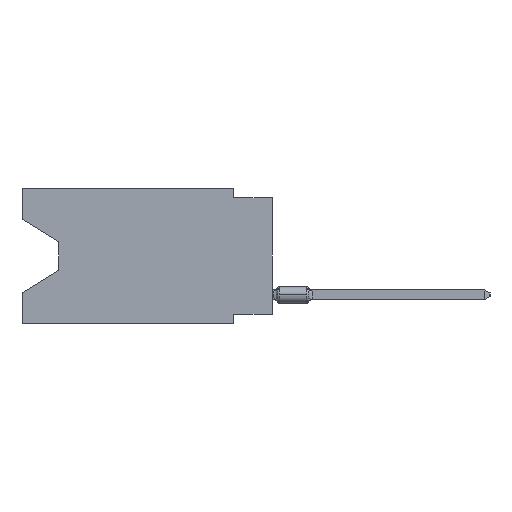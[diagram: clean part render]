
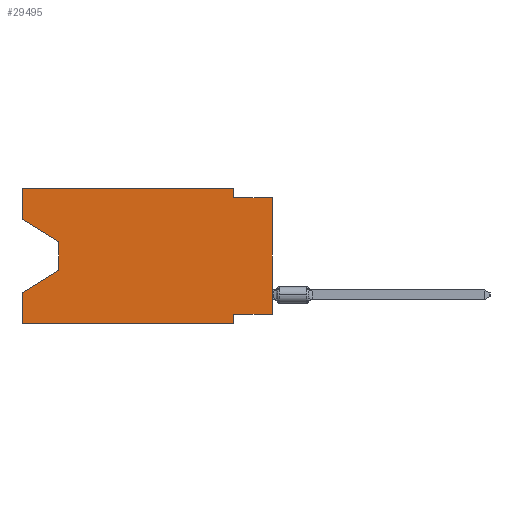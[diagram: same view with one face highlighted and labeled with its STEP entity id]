
A CAD part, left-side view. The second image highlights one B-rep face of the part: STEP entity #29495.
In plain terms, the highlighted planar face has unit normal (-1, 0, 0).
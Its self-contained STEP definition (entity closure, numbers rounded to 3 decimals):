
#459 = LINE ( 'NONE', #22005, #38883 ) ;
#727 = EDGE_CURVE ( 'NONE', #10351, #27550, #41165, .T. ) ;
#1693 = CARTESIAN_POINT ( 'NONE',  ( 0., 0., -0.635 ) ) ;
#2124 = ORIENTED_EDGE ( 'NONE', *, *, #29716, .F. ) ;
#2847 = DIRECTION ( 'NONE',  ( 0., 0., -1. ) ) ;
#3180 = DIRECTION ( 'NONE',  ( 0., -1., 0. ) ) ;
#3705 = EDGE_CURVE ( 'NONE', #16135, #55146, #459, .T. ) ;
#4268 = DIRECTION ( 'NONE',  ( 0., 0., 1. ) ) ;
#4366 = ORIENTED_EDGE ( 'NONE', *, *, #41531, .F. ) ;
#4495 = EDGE_CURVE ( 'NONE', #27789, #14697, #29705, .T. ) ;
#5082 = DIRECTION ( 'NONE',  ( 0., 0., 1. ) ) ;
#6002 = CARTESIAN_POINT ( 'NONE',  ( 0., 16.383, -2.038 ) ) ;
#6176 = DIRECTION ( 'NONE',  ( 0., -1., 0. ) ) ;
#6498 = VERTEX_POINT ( 'NONE', #50728 ) ;
#7904 = CARTESIAN_POINT ( 'NONE',  ( 0., 0., 0. ) ) ;
#8029 = CARTESIAN_POINT ( 'NONE',  ( 0., 16.383, 0. ) ) ;
#8824 = LINE ( 'NONE', #26709, #41561 ) ;
#9826 = VERTEX_POINT ( 'NONE', #49475 ) ;
#10351 = VERTEX_POINT ( 'NONE', #53186 ) ;
#11105 = EDGE_CURVE ( 'NONE', #41352, #16135, #35303, .T. ) ;
#13425 = EDGE_CURVE ( 'NONE', #32368, #14697, #52826, .T. ) ;
#14277 = CARTESIAN_POINT ( 'NONE',  ( 0., 16.383, 0. ) ) ;
#14690 = CARTESIAN_POINT ( 'NONE',  ( 0., 16.383, -8.89 ) ) ;
#14697 = VERTEX_POINT ( 'NONE', #53657 ) ;
#15270 = EDGE_CURVE ( 'NONE', #44979, #41352, #35899, .T. ) ;
#15278 = VECTOR ( 'NONE', #31653, 1000. ) ;
#15598 = LINE ( 'NONE', #8029, #26153 ) ;
#15712 = CARTESIAN_POINT ( 'NONE',  ( 0., 2.54, -8.89 ) ) ;
#16135 = VERTEX_POINT ( 'NONE', #48827 ) ;
#16492 = VECTOR ( 'NONE', #44002, 1000. ) ;
#16639 = EDGE_CURVE ( 'NONE', #6498, #9826, #49581, .T. ) ;
#17535 = DIRECTION ( 'NONE',  ( 0., 0.855, -0.519 ) ) ;
#18446 = PLANE ( 'NONE',  #30715 ) ;
#19275 = DIRECTION ( 'NONE',  ( 1., 0., 0. ) ) ;
#19652 = ORIENTED_EDGE ( 'NONE', *, *, #13425, .F. ) ;
#22005 = CARTESIAN_POINT ( 'NONE',  ( 0., 13.97, -5.385 ) ) ;
#23221 = LINE ( 'NONE', #27414, #32297 ) ;
#25276 = ORIENTED_EDGE ( 'NONE', *, *, #4495, .T. ) ;
#26149 = DIRECTION ( 'NONE',  ( 0., 1., 0. ) ) ;
#26153 = VECTOR ( 'NONE', #30390, 1000. ) ;
#26158 = CARTESIAN_POINT ( 'NONE',  ( 0., 16.383, -6.852 ) ) ;
#26709 = CARTESIAN_POINT ( 'NONE',  ( 0., 0., -8.255 ) ) ;
#27172 = VERTEX_POINT ( 'NONE', #50651 ) ;
#27414 = CARTESIAN_POINT ( 'NONE',  ( 0., 2.54, 0. ) ) ;
#27550 = VERTEX_POINT ( 'NONE', #37206 ) ;
#27644 = FACE_OUTER_BOUND ( 'NONE', #46805, .T. ) ;
#27789 = VERTEX_POINT ( 'NONE', #36030 ) ;
#29495 = ADVANCED_FACE ( 'NONE', ( #27644 ), #18446, .F. ) ;
#29705 = LINE ( 'NONE', #7904, #40766 ) ;
#29716 = EDGE_CURVE ( 'NONE', #44979, #6498, #15598, .T. ) ;
#30390 = DIRECTION ( 'NONE',  ( 0., 0., 1. ) ) ;
#30715 = AXIS2_PLACEMENT_3D ( 'NONE', #44951, #19275, #35748 ) ;
#31315 = LINE ( 'NONE', #14277, #38587 ) ;
#31653 = DIRECTION ( 'NONE',  ( 0., 0., -1. ) ) ;
#31728 = DIRECTION ( 'NONE',  ( 0., -1., 0. ) ) ;
#32297 = VECTOR ( 'NONE', #44177, 1000. ) ;
#32368 = VERTEX_POINT ( 'NONE', #46707 ) ;
#33383 = VECTOR ( 'NONE', #2847, 1000. ) ;
#35040 = ORIENTED_EDGE ( 'NONE', *, *, #15270, .T. ) ;
#35303 = LINE ( 'NONE', #52060, #15278 ) ;
#35748 = DIRECTION ( 'NONE',  ( 0., 0., -1. ) ) ;
#35899 = LINE ( 'NONE', #6002, #16492 ) ;
#36030 = CARTESIAN_POINT ( 'NONE',  ( 0., 0., -8.255 ) ) ;
#36966 = ORIENTED_EDGE ( 'NONE', *, *, #37286, .T. ) ;
#37081 = ORIENTED_EDGE ( 'NONE', *, *, #16639, .F. ) ;
#37206 = CARTESIAN_POINT ( 'NONE',  ( 0., 2.54, -8.89 ) ) ;
#37286 = EDGE_CURVE ( 'NONE', #27172, #27550, #52958, .T. ) ;
#38587 = VECTOR ( 'NONE', #5082, 1000. ) ;
#38883 = VECTOR ( 'NONE', #17535, 1000. ) ;
#39268 = VECTOR ( 'NONE', #31728, 1000. ) ;
#39593 = VECTOR ( 'NONE', #6176, 1000. ) ;
#40625 = ORIENTED_EDGE ( 'NONE', *, *, #727, .F. ) ;
#40766 = VECTOR ( 'NONE', #4268, 1000. ) ;
#41165 = LINE ( 'NONE', #15712, #33383 ) ;
#41352 = VERTEX_POINT ( 'NONE', #51459 ) ;
#41515 = EDGE_CURVE ( 'NONE', #27172, #55146, #31315, .T. ) ;
#41531 = EDGE_CURVE ( 'NONE', #9826, #32368, #23221, .T. ) ;
#41561 = VECTOR ( 'NONE', #26149, 1000. ) ;
#41757 = ORIENTED_EDGE ( 'NONE', *, *, #3705, .T. ) ;
#44002 = DIRECTION ( 'NONE',  ( 0., -0.855, -0.519 ) ) ;
#44177 = DIRECTION ( 'NONE',  ( 0., 0., -1. ) ) ;
#44632 = CARTESIAN_POINT ( 'NONE',  ( 0., 16.383, -2.038 ) ) ;
#44951 = CARTESIAN_POINT ( 'NONE',  ( 0., 16.383, 0. ) ) ;
#44979 = VERTEX_POINT ( 'NONE', #44632 ) ;
#45644 = CARTESIAN_POINT ( 'NONE',  ( 0., 16.383, 0. ) ) ;
#46707 = CARTESIAN_POINT ( 'NONE',  ( 0., 2.54, -0.635 ) ) ;
#46805 = EDGE_LOOP ( 'NONE', ( #35040, #51783, #41757, #49838, #36966, #40625, #53231, #25276, #19652, #4366, #37081, #2124 ) ) ;
#48827 = CARTESIAN_POINT ( 'NONE',  ( 0., 13.97, -5.385 ) ) ;
#49475 = CARTESIAN_POINT ( 'NONE',  ( 0., 2.54, 0. ) ) ;
#49581 = LINE ( 'NONE', #45644, #53055 ) ;
#49838 = ORIENTED_EDGE ( 'NONE', *, *, #41515, .F. ) ;
#50651 = CARTESIAN_POINT ( 'NONE',  ( 0., 16.383, -8.89 ) ) ;
#50728 = CARTESIAN_POINT ( 'NONE',  ( 0., 16.383, 0. ) ) ;
#51459 = CARTESIAN_POINT ( 'NONE',  ( 0., 13.97, -3.505 ) ) ;
#51783 = ORIENTED_EDGE ( 'NONE', *, *, #11105, .T. ) ;
#52060 = CARTESIAN_POINT ( 'NONE',  ( 0., 13.97, -3.505 ) ) ;
#52826 = LINE ( 'NONE', #1693, #39593 ) ;
#52958 = LINE ( 'NONE', #14690, #39268 ) ;
#53055 = VECTOR ( 'NONE', #3180, 1000. ) ;
#53186 = CARTESIAN_POINT ( 'NONE',  ( 0., 2.54, -8.255 ) ) ;
#53231 = ORIENTED_EDGE ( 'NONE', *, *, #53976, .F. ) ;
#53657 = CARTESIAN_POINT ( 'NONE',  ( 0., 0., -0.635 ) ) ;
#53976 = EDGE_CURVE ( 'NONE', #27789, #10351, #8824, .T. ) ;
#55146 = VERTEX_POINT ( 'NONE', #26158 ) ;
